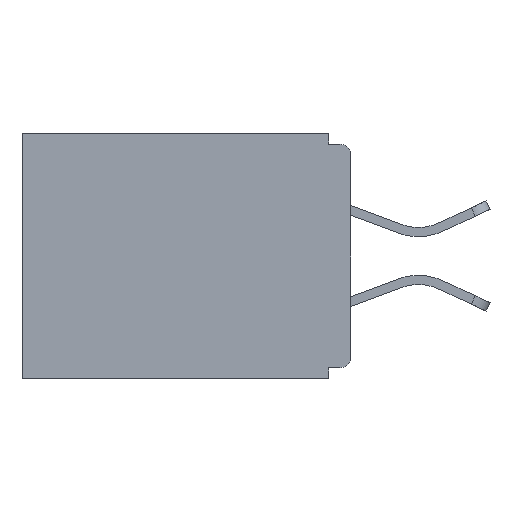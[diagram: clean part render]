
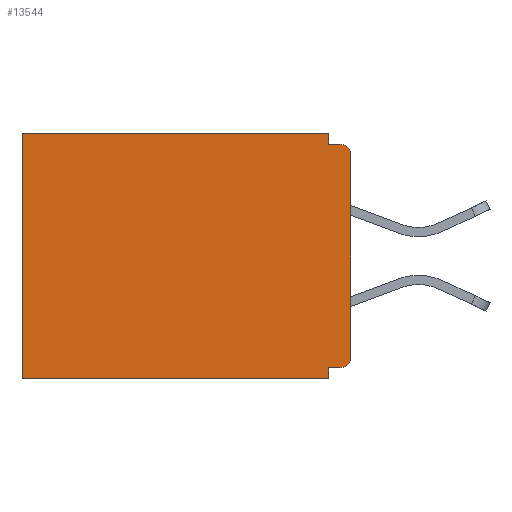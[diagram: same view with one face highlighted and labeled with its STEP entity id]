
A CAD part, left-side view. The second image highlights one B-rep face of the part: STEP entity #13544.
In plain terms, the highlighted planar face has unit normal (-1, 0, 0).
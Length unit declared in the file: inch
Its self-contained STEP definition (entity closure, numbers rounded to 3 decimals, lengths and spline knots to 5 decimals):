
#75 = VERTEX_POINT ( 'NONE', #14434 ) ;
#1274 = EDGE_CURVE ( 'NONE', #17709, #6472, #5448, .T. ) ;
#1517 = VECTOR ( 'NONE', #4620, 39.37008 ) ;
#1558 = EDGE_CURVE ( 'NONE', #13462, #7845, #20874, .T. ) ;
#1811 = CARTESIAN_POINT ( 'NONE',  ( 0.298, 0.015, -0.313 ) ) ;
#2050 = CARTESIAN_POINT ( 'NONE',  ( 0.298, 0., -0.015 ) ) ;
#2819 = VECTOR ( 'NONE', #4935, 39.37008 ) ;
#3078 = CARTESIAN_POINT ( 'NONE',  ( 0.298, 0.015, -0.015 ) ) ;
#3437 = VECTOR ( 'NONE', #14116, 39.37008 ) ;
#3566 = VECTOR ( 'NONE', #9866, 39.37008 ) ;
#3608 = EDGE_CURVE ( 'NONE', #7766, #7845, #14023, .T. ) ;
#3979 = CARTESIAN_POINT ( 'NONE',  ( 0.298, 0.46, 0. ) ) ;
#4383 = CARTESIAN_POINT ( 'NONE',  ( 0.298, 0., -0.03 ) ) ;
#4564 = VECTOR ( 'NONE', #5136, 39.37008 ) ;
#4620 = DIRECTION ( 'NONE',  ( 0., 0., -1. ) ) ;
#4743 = ORIENTED_EDGE ( 'NONE', *, *, #1558, .T. ) ;
#4935 = DIRECTION ( 'NONE',  ( 0., 0., -1. ) ) ;
#5136 = DIRECTION ( 'NONE',  ( 0., -1., 0. ) ) ;
#5383 = LINE ( 'NONE', #9704, #2819 ) ;
#5448 = CIRCLE ( 'NONE', #20314, 0.015 ) ;
#5468 = ORIENTED_EDGE ( 'NONE', *, *, #11313, .T. ) ;
#5595 = DIRECTION ( 'NONE',  ( 0., 0., -1. ) ) ;
#6050 = CARTESIAN_POINT ( 'NONE',  ( 0.298, 0.031, -0.343 ) ) ;
#6251 = CARTESIAN_POINT ( 'NONE',  ( 0.298, 0., -0.343 ) ) ;
#6262 = ORIENTED_EDGE ( 'NONE', *, *, #3608, .F. ) ;
#6472 = VERTEX_POINT ( 'NONE', #3078 ) ;
#6893 = CARTESIAN_POINT ( 'NONE',  ( 0.298, 0.031, 0. ) ) ;
#7618 = VERTEX_POINT ( 'NONE', #18089 ) ;
#7637 = CIRCLE ( 'NONE', #15036, 0.015 ) ;
#7693 = CARTESIAN_POINT ( 'NONE',  ( 0.298, 0.031, -0.328 ) ) ;
#7766 = VERTEX_POINT ( 'NONE', #6050 ) ;
#7845 = VERTEX_POINT ( 'NONE', #18856 ) ;
#7858 = DIRECTION ( 'NONE',  ( 0., 1., 0. ) ) ;
#7911 = EDGE_CURVE ( 'NONE', #17709, #7618, #22694, .T. ) ;
#8057 = CARTESIAN_POINT ( 'NONE',  ( 0.298, 0., 0. ) ) ;
#8140 = CARTESIAN_POINT ( 'NONE',  ( 0.298, 0., -0.328 ) ) ;
#8192 = ORIENTED_EDGE ( 'NONE', *, *, #1274, .T. ) ;
#9704 = CARTESIAN_POINT ( 'NONE',  ( 0.298, 0.031, -0.343 ) ) ;
#9771 = EDGE_CURVE ( 'NONE', #16228, #7766, #12202, .T. ) ;
#9849 = DIRECTION ( 'NONE',  ( 0., 0., -1. ) ) ;
#9866 = DIRECTION ( 'NONE',  ( 0., 0., -1. ) ) ;
#10367 = VECTOR ( 'NONE', #7858, 39.37008 ) ;
#10709 = CARTESIAN_POINT ( 'NONE',  ( 0.298, 0.46, 0. ) ) ;
#11313 = EDGE_CURVE ( 'NONE', #15558, #7618, #7637, .T. ) ;
#11659 = EDGE_CURVE ( 'NONE', #17935, #75, #5383, .T. ) ;
#11773 = CARTESIAN_POINT ( 'NONE',  ( 0.298, 0.031, -0.343 ) ) ;
#11780 = ORIENTED_EDGE ( 'NONE', *, *, #7911, .F. ) ;
#12075 = LINE ( 'NONE', #14932, #10367 ) ;
#12202 = LINE ( 'NONE', #11773, #1517 ) ;
#12937 = EDGE_CURVE ( 'NONE', #15558, #16228, #18335, .T. ) ;
#12972 = VECTOR ( 'NONE', #13896, 39.37008 ) ;
#13462 = VERTEX_POINT ( 'NONE', #3979 ) ;
#13544 = ADVANCED_FACE ( 'NONE', ( #16626 ), #16947, .F. ) ;
#13857 = ORIENTED_EDGE ( 'NONE', *, *, #14665, .T. ) ;
#13896 = DIRECTION ( 'NONE',  ( 0., 1., 0. ) ) ;
#14023 = LINE ( 'NONE', #6251, #18519 ) ;
#14116 = DIRECTION ( 'NONE',  ( 0., 0., -1. ) ) ;
#14434 = CARTESIAN_POINT ( 'NONE',  ( 0.298, 0.031, -0.015 ) ) ;
#14665 = EDGE_CURVE ( 'NONE', #17935, #13462, #12075, .T. ) ;
#14841 = ORIENTED_EDGE ( 'NONE', *, *, #19136, .F. ) ;
#14932 = CARTESIAN_POINT ( 'NONE',  ( 0.298, 0., 0. ) ) ;
#15036 = AXIS2_PLACEMENT_3D ( 'NONE', #1811, #17931, #5595 ) ;
#15077 = ORIENTED_EDGE ( 'NONE', *, *, #9771, .F. ) ;
#15292 = DIRECTION ( 'NONE',  ( 0., 1., 0. ) ) ;
#15295 = DIRECTION ( 'NONE',  ( 0., 0., -1. ) ) ;
#15558 = VERTEX_POINT ( 'NONE', #21466 ) ;
#15820 = LINE ( 'NONE', #2050, #4564 ) ;
#16228 = VERTEX_POINT ( 'NONE', #7693 ) ;
#16626 = FACE_OUTER_BOUND ( 'NONE', #23327, .T. ) ;
#16820 = ORIENTED_EDGE ( 'NONE', *, *, #11659, .F. ) ;
#16873 = DIRECTION ( 'NONE',  ( 1., 0., 0. ) ) ;
#16947 = PLANE ( 'NONE',  #22626 ) ;
#17080 = ORIENTED_EDGE ( 'NONE', *, *, #12937, .F. ) ;
#17709 = VERTEX_POINT ( 'NONE', #4383 ) ;
#17931 = DIRECTION ( 'NONE',  ( -1., 0., 0. ) ) ;
#17935 = VERTEX_POINT ( 'NONE', #6893 ) ;
#18089 = CARTESIAN_POINT ( 'NONE',  ( 0.298, 0., -0.313 ) ) ;
#18335 = LINE ( 'NONE', #8140, #12972 ) ;
#18519 = VECTOR ( 'NONE', #15292, 39.37008 ) ;
#18856 = CARTESIAN_POINT ( 'NONE',  ( 0.298, 0.46, -0.343 ) ) ;
#19136 = EDGE_CURVE ( 'NONE', #75, #6472, #15820, .T. ) ;
#20314 = AXIS2_PLACEMENT_3D ( 'NONE', #22533, #20638, #9849 ) ;
#20638 = DIRECTION ( 'NONE',  ( -1., 0., 0. ) ) ;
#20656 = CARTESIAN_POINT ( 'NONE',  ( 0.298, 0., 0. ) ) ;
#20874 = LINE ( 'NONE', #10709, #3437 ) ;
#21466 = CARTESIAN_POINT ( 'NONE',  ( 0.298, 0.015, -0.328 ) ) ;
#22533 = CARTESIAN_POINT ( 'NONE',  ( 0.298, 0.015, -0.03 ) ) ;
#22626 = AXIS2_PLACEMENT_3D ( 'NONE', #8057, #16873, #15295 ) ;
#22694 = LINE ( 'NONE', #20656, #3566 ) ;
#23327 = EDGE_LOOP ( 'NONE', ( #8192, #14841, #16820, #13857, #4743, #6262, #15077, #17080, #5468, #11780 ) ) ;
